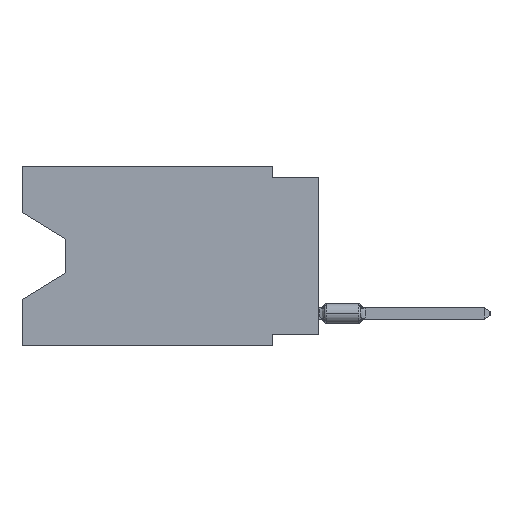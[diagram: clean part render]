
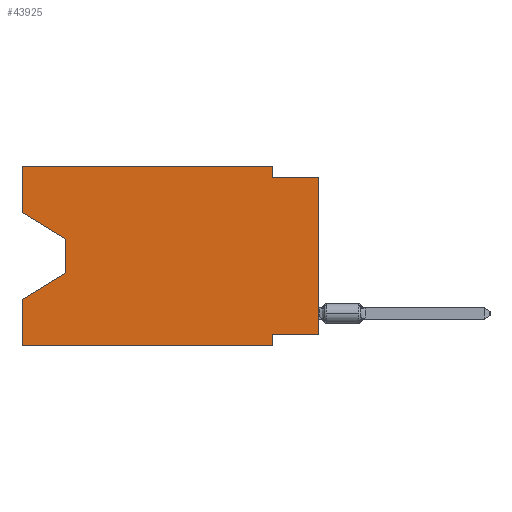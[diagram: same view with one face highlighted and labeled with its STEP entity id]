
A CAD part, left-side view. The second image highlights one B-rep face of the part: STEP entity #43925.
In plain terms, the highlighted planar face has unit normal (-1, 0, 0).
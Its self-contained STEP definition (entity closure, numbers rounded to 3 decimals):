
#199 = DIRECTION ( 'NONE',  ( 0., -1., 0. ) ) ;
#294 = VERTEX_POINT ( 'NONE', #24394 ) ;
#1178 = CARTESIAN_POINT ( 'NONE',  ( 0., 0., -9.271 ) ) ;
#1505 = ORIENTED_EDGE ( 'NONE', *, *, #25328, .F. ) ;
#1586 = CARTESIAN_POINT ( 'NONE',  ( 0., 13.97, -4.013 ) ) ;
#2251 = EDGE_CURVE ( 'NONE', #8196, #46879, #25175, .T. ) ;
#2307 = DIRECTION ( 'NONE',  ( 0., 0., -1. ) ) ;
#2589 = VERTEX_POINT ( 'NONE', #49523 ) ;
#2687 = ORIENTED_EDGE ( 'NONE', *, *, #25411, .T. ) ;
#2784 = VECTOR ( 'NONE', #38587, 1000. ) ;
#3161 = CARTESIAN_POINT ( 'NONE',  ( 0., 16.383, -9.906 ) ) ;
#4027 = LINE ( 'NONE', #7749, #17367 ) ;
#4201 = VERTEX_POINT ( 'NONE', #32243 ) ;
#4528 = EDGE_CURVE ( 'NONE', #8196, #49181, #34620, .T. ) ;
#5577 = EDGE_CURVE ( 'NONE', #19951, #46879, #37026, .T. ) ;
#6076 = ORIENTED_EDGE ( 'NONE', *, *, #35858, .F. ) ;
#6731 = VECTOR ( 'NONE', #7625, 1000. ) ;
#7116 = CARTESIAN_POINT ( 'NONE',  ( 0., 2.54, -9.271 ) ) ;
#7294 = CARTESIAN_POINT ( 'NONE',  ( 0., 16.383, 0. ) ) ;
#7625 = DIRECTION ( 'NONE',  ( 0., -0.855, -0.519 ) ) ;
#7749 = CARTESIAN_POINT ( 'NONE',  ( 0., 0., -0.635 ) ) ;
#8169 = VECTOR ( 'NONE', #41604, 1000. ) ;
#8196 = VERTEX_POINT ( 'NONE', #3161 ) ;
#9029 = ORIENTED_EDGE ( 'NONE', *, *, #24141, .F. ) ;
#9207 = ORIENTED_EDGE ( 'NONE', *, *, #16640, .F. ) ;
#10408 = DIRECTION ( 'NONE',  ( 0., 0., 1. ) ) ;
#11092 = LINE ( 'NONE', #27326, #6731 ) ;
#11563 = VECTOR ( 'NONE', #38078, 1000. ) ;
#12718 = CARTESIAN_POINT ( 'NONE',  ( 0., 13.97, -4.013 ) ) ;
#12726 = VERTEX_POINT ( 'NONE', #13626 ) ;
#13105 = CARTESIAN_POINT ( 'NONE',  ( 0., 16.383, -2.546 ) ) ;
#13188 = CARTESIAN_POINT ( 'NONE',  ( 0., 2.54, -9.906 ) ) ;
#13626 = CARTESIAN_POINT ( 'NONE',  ( 0., 2.54, 0. ) ) ;
#13936 = EDGE_CURVE ( 'NONE', #4201, #49181, #33400, .T. ) ;
#14159 = VERTEX_POINT ( 'NONE', #7294 ) ;
#14385 = CARTESIAN_POINT ( 'NONE',  ( 0., 16.383, 0. ) ) ;
#14482 = VECTOR ( 'NONE', #199, 1000. ) ;
#14661 = EDGE_CURVE ( 'NONE', #52022, #4201, #45403, .T. ) ;
#16640 = EDGE_CURVE ( 'NONE', #2589, #19951, #41843, .T. ) ;
#17181 = DIRECTION ( 'NONE',  ( 0., 0., 1. ) ) ;
#17367 = VECTOR ( 'NONE', #44147, 1000. ) ;
#17439 = DIRECTION ( 'NONE',  ( 0., 0., 1. ) ) ;
#18135 = CARTESIAN_POINT ( 'NONE',  ( 0., 2.54, 0. ) ) ;
#19764 = ORIENTED_EDGE ( 'NONE', *, *, #32455, .F. ) ;
#19951 = VERTEX_POINT ( 'NONE', #7116 ) ;
#20372 = LINE ( 'NONE', #50082, #24467 ) ;
#21016 = CARTESIAN_POINT ( 'NONE',  ( 0., 0., -0.635 ) ) ;
#21698 = LINE ( 'NONE', #37653, #26176 ) ;
#23307 = ORIENTED_EDGE ( 'NONE', *, *, #14661, .T. ) ;
#23465 = VECTOR ( 'NONE', #41000, 1000. ) ;
#23978 = ORIENTED_EDGE ( 'NONE', *, *, #5577, .F. ) ;
#24141 = EDGE_CURVE ( 'NONE', #12726, #294, #30357, .T. ) ;
#24394 = CARTESIAN_POINT ( 'NONE',  ( 0., 2.54, -0.635 ) ) ;
#24467 = VECTOR ( 'NONE', #17181, 1000. ) ;
#24878 = LINE ( 'NONE', #49548, #8169 ) ;
#25175 = LINE ( 'NONE', #36626, #14482 ) ;
#25328 = EDGE_CURVE ( 'NONE', #27463, #14159, #20372, .T. ) ;
#25411 = EDGE_CURVE ( 'NONE', #2589, #39298, #21698, .T. ) ;
#26176 = VECTOR ( 'NONE', #17439, 1000. ) ;
#26359 = VECTOR ( 'NONE', #45584, 1000. ) ;
#27326 = CARTESIAN_POINT ( 'NONE',  ( 0., 16.383, -2.546 ) ) ;
#27463 = VERTEX_POINT ( 'NONE', #13105 ) ;
#27995 = ORIENTED_EDGE ( 'NONE', *, *, #2251, .T. ) ;
#29203 = DIRECTION ( 'NONE',  ( 0., 0., -1. ) ) ;
#29386 = CARTESIAN_POINT ( 'NONE',  ( 0., 13.97, -5.893 ) ) ;
#29635 = AXIS2_PLACEMENT_3D ( 'NONE', #31009, #46404, #2307 ) ;
#30357 = LINE ( 'NONE', #18135, #11563 ) ;
#30551 = VECTOR ( 'NONE', #29203, 1000. ) ;
#31009 = CARTESIAN_POINT ( 'NONE',  ( 0., 16.383, 0. ) ) ;
#31497 = CARTESIAN_POINT ( 'NONE',  ( 0., 16.383, -7.36 ) ) ;
#32243 = CARTESIAN_POINT ( 'NONE',  ( 0., 13.97, -5.893 ) ) ;
#32455 = EDGE_CURVE ( 'NONE', #294, #39298, #4027, .T. ) ;
#33400 = LINE ( 'NONE', #29386, #26359 ) ;
#34521 = EDGE_LOOP ( 'NONE', ( #38350, #23307, #36937, #50996, #27995, #23978, #9207, #2687, #19764, #9029, #6076, #1505 ) ) ;
#34620 = LINE ( 'NONE', #14385, #49550 ) ;
#34755 = PLANE ( 'NONE',  #29635 ) ;
#35858 = EDGE_CURVE ( 'NONE', #14159, #12726, #24878, .T. ) ;
#36626 = CARTESIAN_POINT ( 'NONE',  ( 0., 16.383, -9.906 ) ) ;
#36937 = ORIENTED_EDGE ( 'NONE', *, *, #13936, .T. ) ;
#37026 = LINE ( 'NONE', #44960, #23465 ) ;
#37653 = CARTESIAN_POINT ( 'NONE',  ( 0., 0., 0. ) ) ;
#38078 = DIRECTION ( 'NONE',  ( 0., 0., -1. ) ) ;
#38350 = ORIENTED_EDGE ( 'NONE', *, *, #50533, .T. ) ;
#38587 = DIRECTION ( 'NONE',  ( 0., 1., 0. ) ) ;
#39298 = VERTEX_POINT ( 'NONE', #21016 ) ;
#41000 = DIRECTION ( 'NONE',  ( 0., 0., -1. ) ) ;
#41604 = DIRECTION ( 'NONE',  ( 0., -1., 0. ) ) ;
#41843 = LINE ( 'NONE', #1178, #2784 ) ;
#42705 = FACE_OUTER_BOUND ( 'NONE', #34521, .T. ) ;
#43925 = ADVANCED_FACE ( 'NONE', ( #42705 ), #34755, .F. ) ;
#44147 = DIRECTION ( 'NONE',  ( 0., -1., 0. ) ) ;
#44960 = CARTESIAN_POINT ( 'NONE',  ( 0., 2.54, -9.906 ) ) ;
#45403 = LINE ( 'NONE', #12718, #30551 ) ;
#45584 = DIRECTION ( 'NONE',  ( 0., 0.855, -0.519 ) ) ;
#46404 = DIRECTION ( 'NONE',  ( 1., 0., 0. ) ) ;
#46879 = VERTEX_POINT ( 'NONE', #13188 ) ;
#49181 = VERTEX_POINT ( 'NONE', #31497 ) ;
#49523 = CARTESIAN_POINT ( 'NONE',  ( 0., 0., -9.271 ) ) ;
#49548 = CARTESIAN_POINT ( 'NONE',  ( 0., 16.383, 0. ) ) ;
#49550 = VECTOR ( 'NONE', #10408, 1000. ) ;
#50082 = CARTESIAN_POINT ( 'NONE',  ( 0., 16.383, 0. ) ) ;
#50533 = EDGE_CURVE ( 'NONE', #27463, #52022, #11092, .T. ) ;
#50996 = ORIENTED_EDGE ( 'NONE', *, *, #4528, .F. ) ;
#52022 = VERTEX_POINT ( 'NONE', #1586 ) ;
